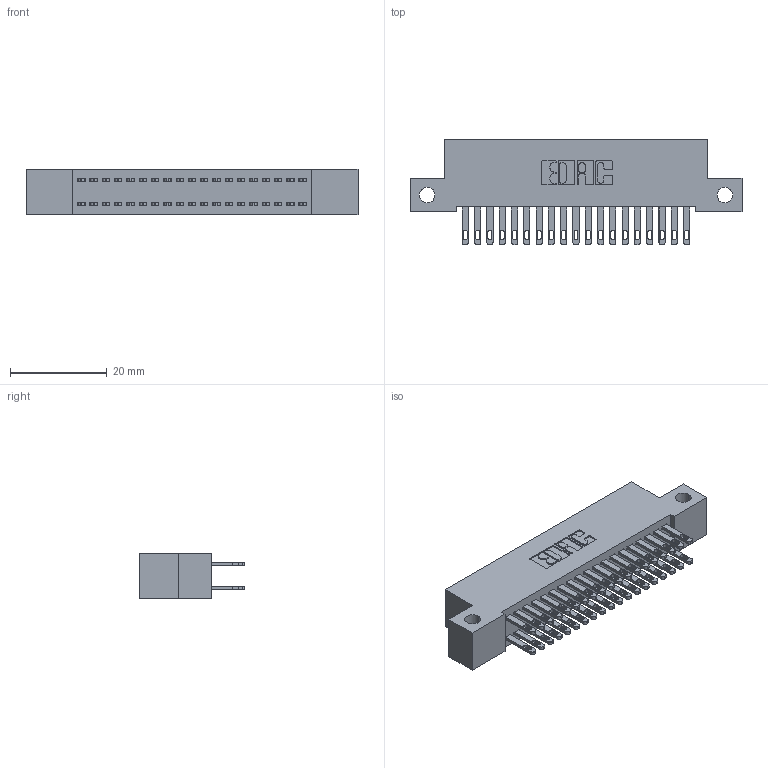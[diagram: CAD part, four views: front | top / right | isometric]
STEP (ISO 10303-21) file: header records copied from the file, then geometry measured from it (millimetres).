
FILE_DESCRIPTION (( 'STEP AP203' ), '1' );
FILE_NAME ('342-038-500-212.STEP', '2019-10-02T14:23:15', ( '' ), ( '' ), 'SwSTEP 2.0', 'SolidWorks 2016', '' );
FILE_SCHEMA (( 'CONFIG_CONTROL_DESIGN' ));
Length unit declared in the file: inch
Products named in the file (3): 342 Part_Side Mount; 345-292-001_345-293-100; 342-038-500-212
Assembly tree (39 placements, depth 2):
  342-038-500-212
    342 Part_Side Mount
    345-292-001_345-293-100  x38
Bounding box: 68.58 x 21.85 x 9.4 mm (x, y, z)
Volume: 6095.2 mm3; surface area: 9558.8 mm2
Topology: 39 solids, 39 shells, 1934 faces, 5885 edges, 3922 vertices
Faces by surface type: plane 1206, cylinder 728
Entity records: 14999 total; most frequent: CARTESIAN_POINT 2510, ORIENTED_EDGE 2446, DIRECTION 2187, EDGE_CURVE 1223, VECTOR 1091, LINE 1091, VERTEX_POINT 814, AXIS2_PLACEMENT_3D 548
